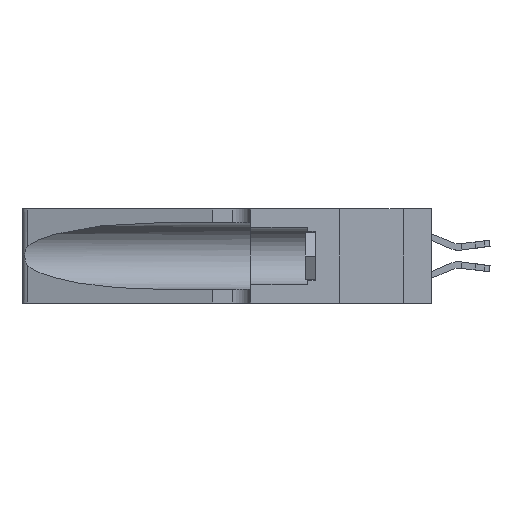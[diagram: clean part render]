
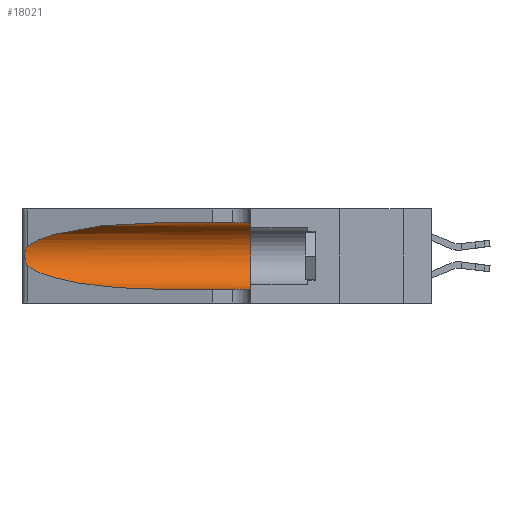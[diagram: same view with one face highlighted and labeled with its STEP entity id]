
A CAD part, left-side view. The second image highlights one B-rep face of the part: STEP entity #18021.
In plain terms, the highlighted cylindrical face has radius 3.308 mm (diameter 6.617 mm), a partial arc.
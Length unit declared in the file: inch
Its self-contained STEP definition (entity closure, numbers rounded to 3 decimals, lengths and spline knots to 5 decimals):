
#63 = LINE ( 'NONE', #12755, #24671 ) ;
#1406 = CARTESIAN_POINT ( 'NONE',  ( 0.26075, 1.23896, 0.178 ) ) ;
#1831 =( BOUNDED_CURVE ( )  B_SPLINE_CURVE ( 3, ( #6598, #30095, #12564, #33045 ),
 .UNSPECIFIED., .F., .T. ) 
 B_SPLINE_CURVE_WITH_KNOTS ( ( 4, 4 ),
 ( 1.5708, 2.84003 ),
 .UNSPECIFIED. ) 
 CURVE ( )  GEOMETRIC_REPRESENTATION_ITEM ( )  RATIONAL_B_SPLINE_CURVE ( ( 1., 0.87, 0.87, 1. ) ) 
 REPRESENTATION_ITEM ( '' )  );
#3109 = DIRECTION ( 'NONE',  ( 0., 1., 0. ) ) ;
#3173 = VERTEX_POINT ( 'NONE', #27522 ) ;
#4457 = CARTESIAN_POINT ( 'NONE',  ( 0.25856, 1.23593, 0.16098 ) ) ;
#4669 = CARTESIAN_POINT ( 'NONE',  ( 0.18966, 0.96281, 0.05475 ) ) ;
#5342 = CARTESIAN_POINT ( 'NONE',  ( 0.1305, 0.35, 0.31525 ) ) ;
#6598 = CARTESIAN_POINT ( 'NONE',  ( 0.1305, 0.72297, 0.31525 ) ) ;
#6970 = VERTEX_POINT ( 'NONE', #34548 ) ;
#7059 = CARTESIAN_POINT ( 'NONE',  ( 0.1305, 1.61858, 0.31525 ) ) ;
#7338 = CARTESIAN_POINT ( 'NONE',  ( 0.25487, 1.22718, 0.22369 ) ) ;
#7360 = DIRECTION ( 'NONE',  ( 0., 0., -1. ) ) ;
#7362 = VERTEX_POINT ( 'NONE', #33487 ) ;
#7461 = CARTESIAN_POINT ( 'NONE',  ( 0.25639, 1.23186, 0.15144 ) ) ;
#7522 = ORIENTED_EDGE ( 'NONE', *, *, #28520, .T. ) ;
#8785 = EDGE_CURVE ( 'NONE', #6970, #37457, #23261, .T. ) ;
#8984 = FACE_OUTER_BOUND ( 'NONE', #14943, .T. ) ;
#10160 = EDGE_CURVE ( 'NONE', #3173, #30787, #31937, .T. ) ;
#10462 = CARTESIAN_POINT ( 'NONE',  ( 0.25487, 1.22718, 0.14631 ) ) ;
#10649 = ORIENTED_EDGE ( 'NONE', *, *, #8785, .T. ) ;
#10910 = CARTESIAN_POINT ( 'NONE',  ( 0.1305, 0.35, 0.05475 ) ) ;
#12564 = CARTESIAN_POINT ( 'NONE',  ( 0.2373, 1.15595, 0.28018 ) ) ;
#12628 = CIRCLE ( 'NONE', #28373, 0.13025 ) ;
#12755 = CARTESIAN_POINT ( 'NONE',  ( 0.1305, 1.61858, 0.05475 ) ) ;
#13308 = CARTESIAN_POINT ( 'NONE',  ( 0.25639, 1.23184, 0.21858 ) ) ;
#13509 = CARTESIAN_POINT ( 'NONE',  ( 0.2373, 1.15595, 0.08982 ) ) ;
#13791 = EDGE_CURVE ( 'NONE', #30787, #32070, #12628, .T. ) ;
#14142 = EDGE_CURVE ( 'NONE', #37457, #7362, #18798, .T. ) ;
#14921 = ORIENTED_EDGE ( 'NONE', *, *, #14142, .T. ) ;
#14943 = EDGE_LOOP ( 'NONE', ( #28676, #10649, #14921, #7522, #18281, #27339 ) ) ;
#15542 = AXIS2_PLACEMENT_3D ( 'NONE', #33925, #22200, #7360 ) ;
#16131 = DIRECTION ( 'NONE',  ( 0., -1., 0. ) ) ;
#16278 = CARTESIAN_POINT ( 'NONE',  ( 0.25854, 1.2359, 0.20912 ) ) ;
#17336 = VECTOR ( 'NONE', #16131, 39.37008 ) ;
#18021 = ADVANCED_FACE ( 'NONE', ( #8984 ), #23735, .F. ) ;
#18281 = ORIENTED_EDGE ( 'NONE', *, *, #13791, .F. ) ;
#18798 =( BOUNDED_CURVE ( )  B_SPLINE_CURVE ( 3, ( #36920, #13509, #4669, #25299 ),
 .UNSPECIFIED., .F., .T. ) 
 B_SPLINE_CURVE_WITH_KNOTS ( ( 4, 4 ),
 ( 3.44316, 4.71239 ),
 .UNSPECIFIED. ) 
 CURVE ( )  GEOMETRIC_REPRESENTATION_ITEM ( )  RATIONAL_B_SPLINE_CURVE ( ( 1., 0.87, 0.87, 1. ) ) 
 REPRESENTATION_ITEM ( '' )  );
#19205 = CARTESIAN_POINT ( 'NONE',  ( 0.26075, 1.23896, 0.19203 ) ) ;
#20866 = CARTESIAN_POINT ( 'NONE',  ( 0.1305, 0.35, 0.185 ) ) ;
#22170 = CARTESIAN_POINT ( 'NONE',  ( 0.26017, 1.23833, 0.17102 ) ) ;
#22200 = DIRECTION ( 'NONE',  ( 0., -1., 0. ) ) ;
#23261 = B_SPLINE_CURVE_WITH_KNOTS ( 'NONE', 3,
 ( #7338, #24977, #13308, #33768, #16278, #36716, #19205, #1406, #22170, #4457, #25099, #7461, #28015, #10462 ),
 .UNSPECIFIED., .F., .F.,
 ( 4, 2, 2, 2, 2, 2, 4 ),
 ( 0., 0.00027, 0.00053, 0.00107, 0.0016, 0.00187, 0.00214 ),
 .UNSPECIFIED. ) ;
#23735 = CYLINDRICAL_SURFACE ( 'NONE', #15542, 0.13025 ) ;
#23796 = DIRECTION ( 'NONE',  ( 0., 0., 1. ) ) ;
#24671 = VECTOR ( 'NONE', #36190, 39.37008 ) ;
#24977 = CARTESIAN_POINT ( 'NONE',  ( 0.25555, 1.22994, 0.2215 ) ) ;
#25099 = CARTESIAN_POINT ( 'NONE',  ( 0.25789, 1.23486, 0.15765 ) ) ;
#25299 = CARTESIAN_POINT ( 'NONE',  ( 0.1305, 0.72297, 0.05475 ) ) ;
#27339 = ORIENTED_EDGE ( 'NONE', *, *, #10160, .F. ) ;
#27522 = CARTESIAN_POINT ( 'NONE',  ( 0.1305, 0.72297, 0.31525 ) ) ;
#28015 = CARTESIAN_POINT ( 'NONE',  ( 0.25555, 1.22993, 0.14849 ) ) ;
#28373 = AXIS2_PLACEMENT_3D ( 'NONE', #20866, #3109, #23796 ) ;
#28520 = EDGE_CURVE ( 'NONE', #7362, #32070, #63, .T. ) ;
#28676 = ORIENTED_EDGE ( 'NONE', *, *, #37037, .T. ) ;
#30095 = CARTESIAN_POINT ( 'NONE',  ( 0.18966, 0.96281, 0.31525 ) ) ;
#30787 = VERTEX_POINT ( 'NONE', #5342 ) ;
#31937 = LINE ( 'NONE', #7059, #17336 ) ;
#32070 = VERTEX_POINT ( 'NONE', #10910 ) ;
#33045 = CARTESIAN_POINT ( 'NONE',  ( 0.25487, 1.22718, 0.22369 ) ) ;
#33487 = CARTESIAN_POINT ( 'NONE',  ( 0.1305, 0.72297, 0.05475 ) ) ;
#33768 = CARTESIAN_POINT ( 'NONE',  ( 0.25787, 1.23484, 0.2124 ) ) ;
#33925 = CARTESIAN_POINT ( 'NONE',  ( 0.1305, 1.61858, 0.185 ) ) ;
#34548 = CARTESIAN_POINT ( 'NONE',  ( 0.25487, 1.22718, 0.22369 ) ) ;
#36190 = DIRECTION ( 'NONE',  ( 0., -1., 0. ) ) ;
#36716 = CARTESIAN_POINT ( 'NONE',  ( 0.26018, 1.23835, 0.19895 ) ) ;
#36920 = CARTESIAN_POINT ( 'NONE',  ( 0.25487, 1.22718, 0.14631 ) ) ;
#37037 = EDGE_CURVE ( 'NONE', #3173, #6970, #1831, .T. ) ;
#37457 = VERTEX_POINT ( 'NONE', #37875 ) ;
#37875 = CARTESIAN_POINT ( 'NONE',  ( 0.25487, 1.22718, 0.14631 ) ) ;
